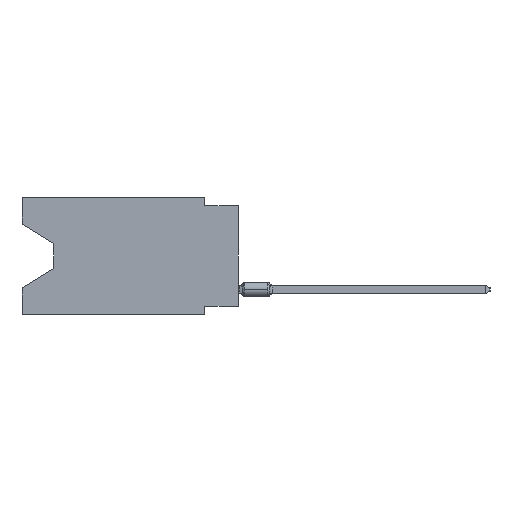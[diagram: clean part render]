
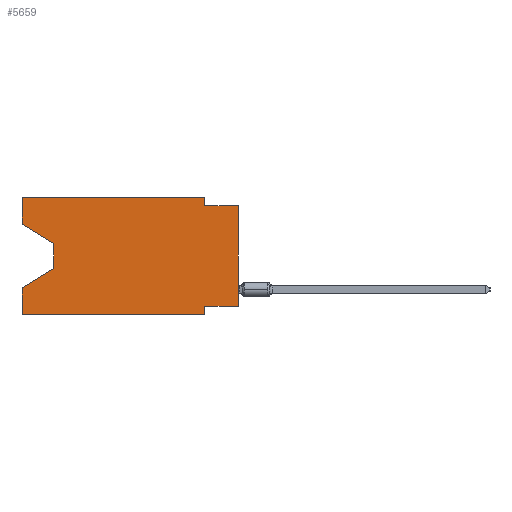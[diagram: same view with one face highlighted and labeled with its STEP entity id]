
A CAD part, left-side view. The second image highlights one B-rep face of the part: STEP entity #5659.
In plain terms, the highlighted planar face has unit normal (-1, 0, 0).
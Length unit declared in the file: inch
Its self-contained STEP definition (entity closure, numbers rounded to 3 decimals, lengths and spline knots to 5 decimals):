
#498 = ORIENTED_EDGE ( 'NONE', *, *, #33949, .T. ) ;
#1001 = VERTEX_POINT ( 'NONE', #25117 ) ;
#1851 = DIRECTION ( 'NONE',  ( 0., 0., 1. ) ) ;
#1864 = DIRECTION ( 'NONE',  ( 0., -1., 0. ) ) ;
#1901 = VERTEX_POINT ( 'NONE', #10020 ) ;
#2035 = EDGE_CURVE ( 'NONE', #8534, #20818, #29729, .T. ) ;
#2500 = VECTOR ( 'NONE', #32022, 39.37008 ) ;
#2660 = CARTESIAN_POINT ( 'NONE',  ( 0., 0.55, -0.138 ) ) ;
#2985 = ORIENTED_EDGE ( 'NONE', *, *, #13860, .F. ) ;
#3493 = VERTEX_POINT ( 'NONE', #19703 ) ;
#3538 = VECTOR ( 'NONE', #35067, 39.37008 ) ;
#3605 = CARTESIAN_POINT ( 'NONE',  ( 0., 0.1, 0. ) ) ;
#3980 = ORIENTED_EDGE ( 'NONE', *, *, #10378, .F. ) ;
#4171 = EDGE_CURVE ( 'NONE', #1001, #34440, #29225, .T. ) ;
#4549 = CARTESIAN_POINT ( 'NONE',  ( 0., 0.645, 0. ) ) ;
#5039 = DIRECTION ( 'NONE',  ( 0., -1., 0. ) ) ;
#5209 = CARTESIAN_POINT ( 'NONE',  ( 0., 0.55, -0.212 ) ) ;
#5659 = ADVANCED_FACE ( 'NONE', ( #19662 ), #31181, .F. ) ;
#5933 = ORIENTED_EDGE ( 'NONE', *, *, #4171, .T. ) ;
#6350 = LINE ( 'NONE', #9029, #8165 ) ;
#7365 = LINE ( 'NONE', #15730, #26946 ) ;
#7629 = DIRECTION ( 'NONE',  ( 0., 0., -1. ) ) ;
#7635 = VECTOR ( 'NONE', #19017, 39.37008 ) ;
#8165 = VECTOR ( 'NONE', #28048, 39.37008 ) ;
#8326 = CARTESIAN_POINT ( 'NONE',  ( 0., 0.1, -0.325 ) ) ;
#8534 = VERTEX_POINT ( 'NONE', #3605 ) ;
#8794 = LINE ( 'NONE', #30298, #16248 ) ;
#9029 = CARTESIAN_POINT ( 'NONE',  ( 0., 0.1, -0.35 ) ) ;
#9263 = EDGE_CURVE ( 'NONE', #9548, #25106, #26717, .T. ) ;
#9548 = VERTEX_POINT ( 'NONE', #14449 ) ;
#9815 = VECTOR ( 'NONE', #33647, 39.37008 ) ;
#9915 = CARTESIAN_POINT ( 'NONE',  ( 0., 0.1, -0.025 ) ) ;
#10020 = CARTESIAN_POINT ( 'NONE',  ( 0., 0.1, -0.35 ) ) ;
#10378 = EDGE_CURVE ( 'NONE', #20818, #34440, #7365, .T. ) ;
#10663 = CARTESIAN_POINT ( 'NONE',  ( 0., 0.645, -0.26975 ) ) ;
#11150 = ORIENTED_EDGE ( 'NONE', *, *, #17166, .F. ) ;
#11199 = LINE ( 'NONE', #27369, #18321 ) ;
#11695 = AXIS2_PLACEMENT_3D ( 'NONE', #12160, #14300, #11973 ) ;
#11961 = CARTESIAN_POINT ( 'NONE',  ( 0., 0.645, 0. ) ) ;
#11973 = DIRECTION ( 'NONE',  ( 0., 0., -1. ) ) ;
#12143 = LINE ( 'NONE', #11961, #9815 ) ;
#12160 = CARTESIAN_POINT ( 'NONE',  ( 0., 0.645, 0. ) ) ;
#12867 = LINE ( 'NONE', #21563, #24638 ) ;
#13660 = LINE ( 'NONE', #2660, #21799 ) ;
#13860 = EDGE_CURVE ( 'NONE', #26766, #25106, #28113, .T. ) ;
#14300 = DIRECTION ( 'NONE',  ( 1., 0., 0. ) ) ;
#14359 = ORIENTED_EDGE ( 'NONE', *, *, #2035, .F. ) ;
#14449 = CARTESIAN_POINT ( 'NONE',  ( 0., 0.55, -0.212 ) ) ;
#15237 = VERTEX_POINT ( 'NONE', #4549 ) ;
#15730 = CARTESIAN_POINT ( 'NONE',  ( 0., 0., -0.025 ) ) ;
#16056 = DIRECTION ( 'NONE',  ( 0., 0.855, -0.519 ) ) ;
#16248 = VECTOR ( 'NONE', #19966, 39.37008 ) ;
#17166 = EDGE_CURVE ( 'NONE', #15237, #8534, #12867, .T. ) ;
#17662 = EDGE_CURVE ( 'NONE', #1001, #25654, #11199, .T. ) ;
#18321 = VECTOR ( 'NONE', #27197, 39.37008 ) ;
#18474 = CARTESIAN_POINT ( 'NONE',  ( 0., 0., -0.025 ) ) ;
#18711 = CARTESIAN_POINT ( 'NONE',  ( 0., 0.1, 0. ) ) ;
#19017 = DIRECTION ( 'NONE',  ( 0., 0., 1. ) ) ;
#19338 = ORIENTED_EDGE ( 'NONE', *, *, #9263, .T. ) ;
#19662 = FACE_OUTER_BOUND ( 'NONE', #28255, .T. ) ;
#19703 = CARTESIAN_POINT ( 'NONE',  ( 0., 0.55, -0.138 ) ) ;
#19966 = DIRECTION ( 'NONE',  ( 0., -1., 0. ) ) ;
#20818 = VERTEX_POINT ( 'NONE', #9915 ) ;
#21143 = CARTESIAN_POINT ( 'NONE',  ( 0., 0.645, 0. ) ) ;
#21375 = CARTESIAN_POINT ( 'NONE',  ( 0., 0.645, -0.08025 ) ) ;
#21563 = CARTESIAN_POINT ( 'NONE',  ( 0., 0.645, 0. ) ) ;
#21799 = VECTOR ( 'NONE', #7629, 39.37008 ) ;
#22304 = ORIENTED_EDGE ( 'NONE', *, *, #24352, .T. ) ;
#24352 = EDGE_CURVE ( 'NONE', #26766, #1901, #8794, .T. ) ;
#24638 = VECTOR ( 'NONE', #5039, 39.37008 ) ;
#24776 = CARTESIAN_POINT ( 'NONE',  ( 0., 0.645, -0.08025 ) ) ;
#25106 = VERTEX_POINT ( 'NONE', #10663 ) ;
#25117 = CARTESIAN_POINT ( 'NONE',  ( 0., 0., -0.325 ) ) ;
#25654 = VERTEX_POINT ( 'NONE', #8326 ) ;
#25901 = ORIENTED_EDGE ( 'NONE', *, *, #26330, .F. ) ;
#26030 = CARTESIAN_POINT ( 'NONE',  ( 0., 0., 0. ) ) ;
#26330 = EDGE_CURVE ( 'NONE', #32626, #15237, #12143, .T. ) ;
#26650 = ORIENTED_EDGE ( 'NONE', *, *, #33281, .T. ) ;
#26717 = LINE ( 'NONE', #5209, #30691 ) ;
#26766 = VERTEX_POINT ( 'NONE', #28403 ) ;
#26946 = VECTOR ( 'NONE', #1864, 39.37008 ) ;
#27197 = DIRECTION ( 'NONE',  ( 0., 1., 0. ) ) ;
#27198 = VECTOR ( 'NONE', #1851, 39.37008 ) ;
#27369 = CARTESIAN_POINT ( 'NONE',  ( 0., 0., -0.325 ) ) ;
#28048 = DIRECTION ( 'NONE',  ( 0., 0., -1. ) ) ;
#28113 = LINE ( 'NONE', #21143, #7635 ) ;
#28255 = EDGE_LOOP ( 'NONE', ( #498, #26650, #19338, #2985, #22304, #34314, #30353, #5933, #3980, #14359, #11150, #25901 ) ) ;
#28403 = CARTESIAN_POINT ( 'NONE',  ( 0., 0.645, -0.35 ) ) ;
#29225 = LINE ( 'NONE', #26030, #27198 ) ;
#29729 = LINE ( 'NONE', #18711, #3538 ) ;
#30298 = CARTESIAN_POINT ( 'NONE',  ( 0., 0.645, -0.35 ) ) ;
#30353 = ORIENTED_EDGE ( 'NONE', *, *, #17662, .F. ) ;
#30691 = VECTOR ( 'NONE', #16056, 39.37008 ) ;
#31181 = PLANE ( 'NONE',  #11695 ) ;
#31675 = LINE ( 'NONE', #21375, #2500 ) ;
#32022 = DIRECTION ( 'NONE',  ( 0., -0.855, -0.519 ) ) ;
#32626 = VERTEX_POINT ( 'NONE', #24776 ) ;
#33281 = EDGE_CURVE ( 'NONE', #3493, #9548, #13660, .T. ) ;
#33647 = DIRECTION ( 'NONE',  ( 0., 0., 1. ) ) ;
#33949 = EDGE_CURVE ( 'NONE', #32626, #3493, #31675, .T. ) ;
#34314 = ORIENTED_EDGE ( 'NONE', *, *, #34709, .F. ) ;
#34440 = VERTEX_POINT ( 'NONE', #18474 ) ;
#34709 = EDGE_CURVE ( 'NONE', #25654, #1901, #6350, .T. ) ;
#35067 = DIRECTION ( 'NONE',  ( 0., 0., -1. ) ) ;
